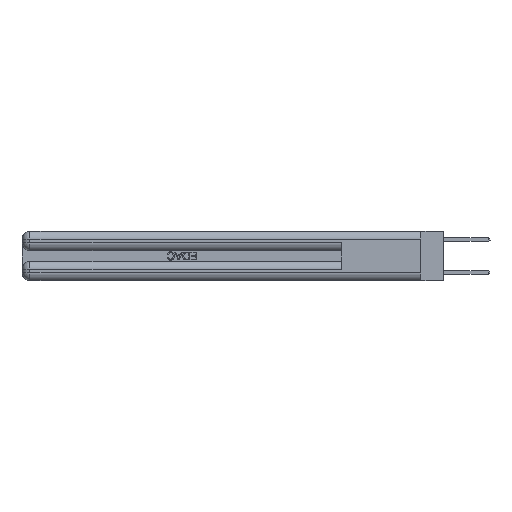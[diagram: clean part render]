
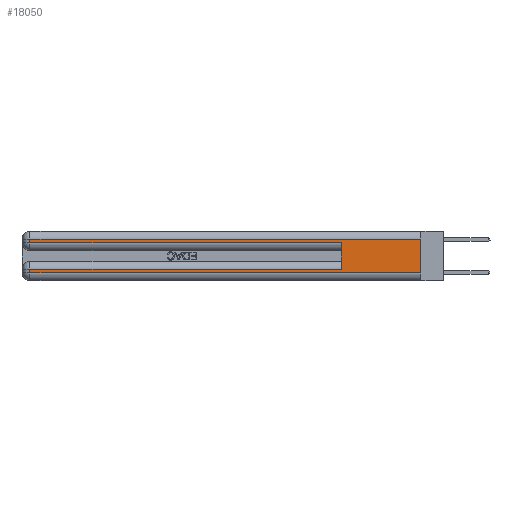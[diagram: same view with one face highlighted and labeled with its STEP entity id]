
A CAD part, left-side view. The second image highlights one B-rep face of the part: STEP entity #18050.
In plain terms, the highlighted planar face has unit normal (-1, 0, 0).
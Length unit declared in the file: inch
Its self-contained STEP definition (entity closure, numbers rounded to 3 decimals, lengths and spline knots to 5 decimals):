
#1922 = EDGE_CURVE ( 'NONE', #3972, #25753, #11688, .T. ) ;
#2200 = CARTESIAN_POINT ( 'NONE',  ( 0., 0.6, 0.285 ) ) ;
#2889 = EDGE_CURVE ( 'NONE', #7524, #12490, #18235, .T. ) ;
#3972 = VERTEX_POINT ( 'NONE', #9839 ) ;
#4864 = CARTESIAN_POINT ( 'NONE',  ( 0., 0., 0.37 ) ) ;
#5766 = AXIS2_PLACEMENT_3D ( 'NONE', #13494, #25988, #11077 ) ;
#5813 = DIRECTION ( 'NONE',  ( 0., 0., 1. ) ) ;
#7028 = EDGE_CURVE ( 'NONE', #12925, #27904, #23891, .T. ) ;
#7063 = ORIENTED_EDGE ( 'NONE', *, *, #28036, .T. ) ;
#7333 = EDGE_CURVE ( 'NONE', #27904, #21801, #16853, .T. ) ;
#7524 = VERTEX_POINT ( 'NONE', #18754 ) ;
#7720 = DIRECTION ( 'NONE',  ( 0., -1., 0. ) ) ;
#8007 = LINE ( 'NONE', #31553, #21267 ) ;
#8201 = DIRECTION ( 'NONE',  ( 0., -1., 0. ) ) ;
#8983 = ORIENTED_EDGE ( 'NONE', *, *, #2889, .F. ) ;
#9203 = DIRECTION ( 'NONE',  ( 0., 1., 0. ) ) ;
#9839 = CARTESIAN_POINT ( 'NONE',  ( 0., 2.94, 0.085 ) ) ;
#10561 = ORIENTED_EDGE ( 'NONE', *, *, #15433, .T. ) ;
#10629 = VECTOR ( 'NONE', #19003, 39.37008 ) ;
#10737 = EDGE_CURVE ( 'NONE', #17413, #21801, #14003, .T. ) ;
#11077 = DIRECTION ( 'NONE',  ( 0., 0., -1. ) ) ;
#11267 = CARTESIAN_POINT ( 'NONE',  ( 0., 2.94, 0.285 ) ) ;
#11633 = VECTOR ( 'NONE', #5813, 39.37008 ) ;
#11688 = LINE ( 'NONE', #21084, #29942 ) ;
#11806 = EDGE_CURVE ( 'NONE', #25753, #12490, #17411, .T. ) ;
#12151 = ORIENTED_EDGE ( 'NONE', *, *, #7333, .T. ) ;
#12490 = VERTEX_POINT ( 'NONE', #20206 ) ;
#12925 = VERTEX_POINT ( 'NONE', #27029 ) ;
#13069 = CARTESIAN_POINT ( 'NONE',  ( 0., 0.6, 0.085 ) ) ;
#13494 = CARTESIAN_POINT ( 'NONE',  ( 0., 0., 0.37 ) ) ;
#14003 = LINE ( 'NONE', #30597, #11633 ) ;
#15266 = ORIENTED_EDGE ( 'NONE', *, *, #11806, .T. ) ;
#15433 = EDGE_CURVE ( 'NONE', #7524, #12925, #24736, .T. ) ;
#16728 = DIRECTION ( 'NONE',  ( 0., 1., 0. ) ) ;
#16853 = LINE ( 'NONE', #30576, #22704 ) ;
#17222 = FACE_OUTER_BOUND ( 'NONE', #21545, .T. ) ;
#17411 = LINE ( 'NONE', #25145, #24042 ) ;
#17413 = VERTEX_POINT ( 'NONE', #13069 ) ;
#18050 = ADVANCED_FACE ( 'NONE', ( #17222 ), #20988, .F. ) ;
#18235 = LINE ( 'NONE', #4864, #24085 ) ;
#18754 = CARTESIAN_POINT ( 'NONE',  ( 0., 0., 0.31 ) ) ;
#19003 = DIRECTION ( 'NONE',  ( 0., 0., -1. ) ) ;
#20079 = CARTESIAN_POINT ( 'NONE',  ( 0., 2.94, 0.06 ) ) ;
#20206 = CARTESIAN_POINT ( 'NONE',  ( 0., 0., 0.06 ) ) ;
#20988 = PLANE ( 'NONE',  #5766 ) ;
#21084 = CARTESIAN_POINT ( 'NONE',  ( 0., 2.94, 0.37 ) ) ;
#21267 = VECTOR ( 'NONE', #16728, 39.37008 ) ;
#21534 = CARTESIAN_POINT ( 'NONE',  ( 0., 2.94, 0.37 ) ) ;
#21545 = EDGE_LOOP ( 'NONE', ( #8983, #10561, #23821, #12151, #26146, #7063, #27700, #15266 ) ) ;
#21801 = VERTEX_POINT ( 'NONE', #2200 ) ;
#22704 = VECTOR ( 'NONE', #8201, 39.37008 ) ;
#23598 = DIRECTION ( 'NONE',  ( 0., 0., -1. ) ) ;
#23821 = ORIENTED_EDGE ( 'NONE', *, *, #7028, .T. ) ;
#23891 = LINE ( 'NONE', #21534, #10629 ) ;
#24042 = VECTOR ( 'NONE', #7720, 39.37008 ) ;
#24085 = VECTOR ( 'NONE', #27325, 39.37008 ) ;
#24736 = LINE ( 'NONE', #31552, #30525 ) ;
#25145 = CARTESIAN_POINT ( 'NONE',  ( 0., 0., 0.06 ) ) ;
#25753 = VERTEX_POINT ( 'NONE', #20079 ) ;
#25988 = DIRECTION ( 'NONE',  ( 1., 0., 0. ) ) ;
#26146 = ORIENTED_EDGE ( 'NONE', *, *, #10737, .F. ) ;
#27029 = CARTESIAN_POINT ( 'NONE',  ( 0., 2.94, 0.31 ) ) ;
#27325 = DIRECTION ( 'NONE',  ( 0., 0., -1. ) ) ;
#27700 = ORIENTED_EDGE ( 'NONE', *, *, #1922, .T. ) ;
#27904 = VERTEX_POINT ( 'NONE', #11267 ) ;
#28036 = EDGE_CURVE ( 'NONE', #17413, #3972, #8007, .T. ) ;
#29942 = VECTOR ( 'NONE', #23598, 39.37008 ) ;
#30525 = VECTOR ( 'NONE', #9203, 39.37008 ) ;
#30576 = CARTESIAN_POINT ( 'NONE',  ( 0., 0., 0.285 ) ) ;
#30597 = CARTESIAN_POINT ( 'NONE',  ( 0., 0.6, 0.145 ) ) ;
#31552 = CARTESIAN_POINT ( 'NONE',  ( 0., 0., 0.31 ) ) ;
#31553 = CARTESIAN_POINT ( 'NONE',  ( 0., 0., 0.085 ) ) ;
